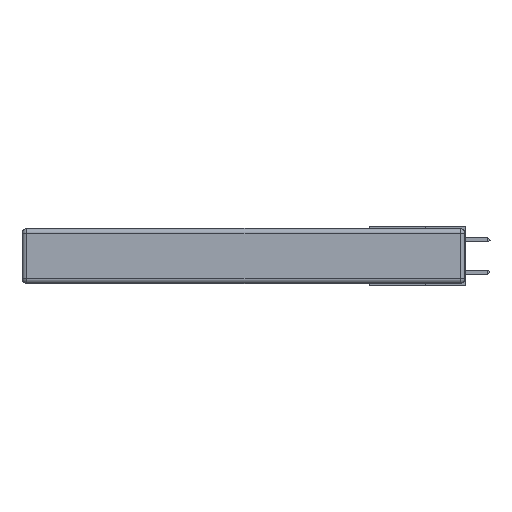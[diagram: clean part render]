
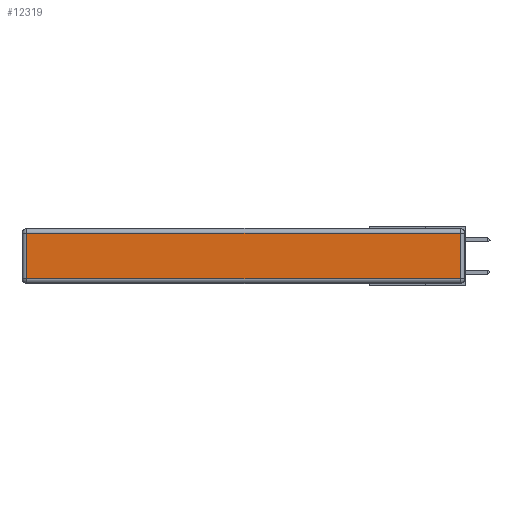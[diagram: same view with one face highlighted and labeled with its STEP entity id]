
A CAD part, left-side view. The second image highlights one B-rep face of the part: STEP entity #12319.
In plain terms, the highlighted planar face has unit normal (-1, 0, 0).
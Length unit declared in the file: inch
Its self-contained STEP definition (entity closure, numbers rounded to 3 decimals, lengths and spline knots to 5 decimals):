
#492 = CARTESIAN_POINT ( 'NONE',  ( 0., 2.72, -0.03 ) ) ;
#860 = VECTOR ( 'NONE', #6000, 39.37008 ) ;
#1283 = LINE ( 'NONE', #3505, #3031 ) ;
#3031 = VECTOR ( 'NONE', #12816, 39.37008 ) ;
#3505 = CARTESIAN_POINT ( 'NONE',  ( 0., 0.03, -0.343 ) ) ;
#3759 = DIRECTION ( 'NONE',  ( 0., 1., 0. ) ) ;
#3910 = EDGE_CURVE ( 'NONE', #15440, #20303, #15781, .T. ) ;
#4002 = VERTEX_POINT ( 'NONE', #13422 ) ;
#4628 = CARTESIAN_POINT ( 'NONE',  ( 0., 0., -0.313 ) ) ;
#4900 = ORIENTED_EDGE ( 'NONE', *, *, #3910, .T. ) ;
#4912 = CARTESIAN_POINT ( 'NONE',  ( 0., 0.03, -0.03 ) ) ;
#5199 = DIRECTION ( 'NONE',  ( 0., -1., 0. ) ) ;
#5841 = AXIS2_PLACEMENT_3D ( 'NONE', #19839, #18056, #10353 ) ;
#6000 = DIRECTION ( 'NONE',  ( 0., 0., -1. ) ) ;
#6771 = CARTESIAN_POINT ( 'NONE',  ( 0., 0.03, -0.313 ) ) ;
#7063 = ORIENTED_EDGE ( 'NONE', *, *, #10431, .T. ) ;
#8157 = EDGE_CURVE ( 'NONE', #20303, #4002, #9516, .T. ) ;
#8760 = PLANE ( 'NONE',  #5841 ) ;
#9294 = LINE ( 'NONE', #4628, #13746 ) ;
#9492 = FACE_OUTER_BOUND ( 'NONE', #18824, .T. ) ;
#9516 = LINE ( 'NONE', #15265, #860 ) ;
#10353 = DIRECTION ( 'NONE',  ( 0., 0., 1. ) ) ;
#10431 = EDGE_CURVE ( 'NONE', #18570, #15440, #1283, .T. ) ;
#11330 = EDGE_CURVE ( 'NONE', #4002, #18570, #9294, .T. ) ;
#11566 = VECTOR ( 'NONE', #3759, 39.37008 ) ;
#11961 = ORIENTED_EDGE ( 'NONE', *, *, #8157, .T. ) ;
#12319 = ADVANCED_FACE ( 'NONE', ( #9492 ), #8760, .T. ) ;
#12816 = DIRECTION ( 'NONE',  ( 0., 0., 1. ) ) ;
#13422 = CARTESIAN_POINT ( 'NONE',  ( 0., 2.72, -0.313 ) ) ;
#13746 = VECTOR ( 'NONE', #5199, 39.37008 ) ;
#15265 = CARTESIAN_POINT ( 'NONE',  ( 0., 2.72, -0.343 ) ) ;
#15440 = VERTEX_POINT ( 'NONE', #4912 ) ;
#15781 = LINE ( 'NONE', #18035, #11566 ) ;
#18035 = CARTESIAN_POINT ( 'NONE',  ( 0., 2.75, -0.03 ) ) ;
#18056 = DIRECTION ( 'NONE',  ( -1., 0., 0. ) ) ;
#18570 = VERTEX_POINT ( 'NONE', #6771 ) ;
#18824 = EDGE_LOOP ( 'NONE', ( #18899, #7063, #4900, #11961 ) ) ;
#18899 = ORIENTED_EDGE ( 'NONE', *, *, #11330, .T. ) ;
#19839 = CARTESIAN_POINT ( 'NONE',  ( 0., 0., -0.343 ) ) ;
#20303 = VERTEX_POINT ( 'NONE', #492 ) ;
